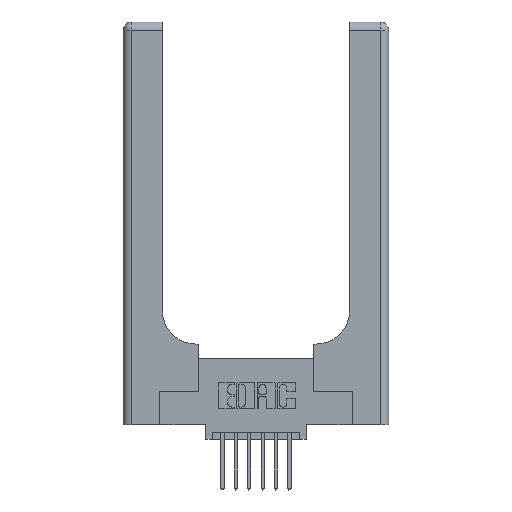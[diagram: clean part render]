
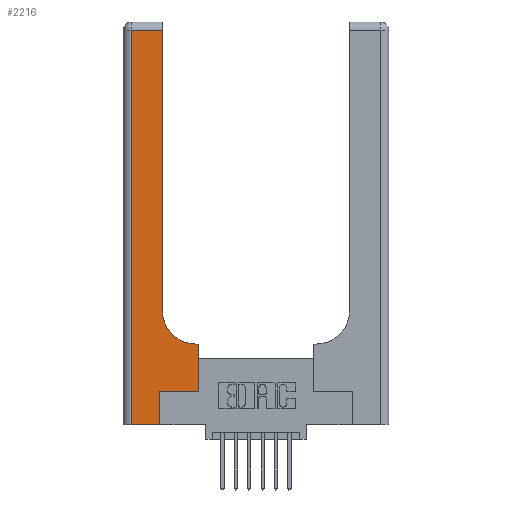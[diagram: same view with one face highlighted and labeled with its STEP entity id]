
A CAD part, top view. The second image highlights one B-rep face of the part: STEP entity #2216.
In plain terms, the highlighted planar face has unit normal (0, 0, 1).
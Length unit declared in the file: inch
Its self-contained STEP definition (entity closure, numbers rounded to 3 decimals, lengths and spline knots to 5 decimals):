
#297 = VECTOR ( 'NONE', #5770, 39.37008 ) ;
#603 = CARTESIAN_POINT ( 'NONE',  ( 0.269, 0., 0.37 ) ) ;
#843 = EDGE_CURVE ( 'NONE', #1696, #10269, #12274, .T. ) ;
#883 = AXIS2_PLACEMENT_3D ( 'NONE', #6288, #6208, #6057 ) ;
#1347 = LINE ( 'NONE', #8570, #10317 ) ;
#1508 = CARTESIAN_POINT ( 'NONE',  ( 0.2915, 0.6, 0.37 ) ) ;
#1696 = VERTEX_POINT ( 'NONE', #8972 ) ;
#1729 = CARTESIAN_POINT ( 'NONE',  ( 0.5415, 0.6, 0.37 ) ) ;
#2173 = AXIS2_PLACEMENT_3D ( 'NONE', #11557, #4662, #12651 ) ;
#2216 = ADVANCED_FACE ( 'NONE', ( #4907 ), #6676, .F. ) ;
#2738 = EDGE_CURVE ( 'NONE', #10291, #11556, #1347, .T. ) ;
#2952 = LINE ( 'NONE', #603, #14740 ) ;
#3196 = ORIENTED_EDGE ( 'NONE', *, *, #8487, .T. ) ;
#3889 = DIRECTION ( 'NONE',  ( -1., 0., 0. ) ) ;
#4345 = LINE ( 'NONE', #14715, #10156 ) ;
#4662 = DIRECTION ( 'NONE',  ( 0., 0., -1. ) ) ;
#4897 = ORIENTED_EDGE ( 'NONE', *, *, #2738, .T. ) ;
#4907 = FACE_OUTER_BOUND ( 'NONE', #8575, .T. ) ;
#5041 = VERTEX_POINT ( 'NONE', #7053 ) ;
#5174 = CARTESIAN_POINT ( 'NONE',  ( 0.5585, 0.6, 0.37 ) ) ;
#5247 = CIRCLE ( 'NONE', #2173, 0.25 ) ;
#5265 = VERTEX_POINT ( 'NONE', #5174 ) ;
#5685 = CARTESIAN_POINT ( 'NONE',  ( 0., 0., 0.37 ) ) ;
#5710 = VERTEX_POINT ( 'NONE', #5905 ) ;
#5770 = DIRECTION ( 'NONE',  ( 1., 0., 0. ) ) ;
#5905 = CARTESIAN_POINT ( 'NONE',  ( 0.2915, 0.85, 0.37 ) ) ;
#5964 = CARTESIAN_POINT ( 'NONE',  ( 0.269, 0., 0.37 ) ) ;
#5968 = DIRECTION ( 'NONE',  ( 0., -1., 0. ) ) ;
#6057 = DIRECTION ( 'NONE',  ( -1., 0., 0. ) ) ;
#6208 = DIRECTION ( 'NONE',  ( 0., 0., -1. ) ) ;
#6288 = CARTESIAN_POINT ( 'NONE',  ( 0., 3., 0.37 ) ) ;
#6676 = PLANE ( 'NONE',  #883 ) ;
#7053 = CARTESIAN_POINT ( 'NONE',  ( 0.06, 2.94, 0.37 ) ) ;
#7256 = VECTOR ( 'NONE', #8825, 39.37008 ) ;
#7663 = CARTESIAN_POINT ( 'NONE',  ( 0.2915, 3., 0.37 ) ) ;
#7739 = ORIENTED_EDGE ( 'NONE', *, *, #9788, .T. ) ;
#7916 = ORIENTED_EDGE ( 'NONE', *, *, #14826, .T. ) ;
#7942 = VECTOR ( 'NONE', #3889, 39.37008 ) ;
#7957 = VERTEX_POINT ( 'NONE', #14883 ) ;
#8397 = EDGE_CURVE ( 'NONE', #8807, #5710, #5247, .T. ) ;
#8431 = ORIENTED_EDGE ( 'NONE', *, *, #10467, .T. ) ;
#8487 = EDGE_CURVE ( 'NONE', #5041, #1696, #9951, .T. ) ;
#8570 = CARTESIAN_POINT ( 'NONE',  ( 0.269, 0.25, 0.37 ) ) ;
#8575 = EDGE_LOOP ( 'NONE', ( #9108, #7916, #3196, #12663, #8431, #4897, #10597, #7739, #14172 ) ) ;
#8655 = DIRECTION ( 'NONE',  ( 1., 0., 0. ) ) ;
#8807 = VERTEX_POINT ( 'NONE', #1729 ) ;
#8825 = DIRECTION ( 'NONE',  ( -1., 0., 0. ) ) ;
#8911 = LINE ( 'NONE', #7663, #11904 ) ;
#8972 = CARTESIAN_POINT ( 'NONE',  ( 0.06, 0., 0.37 ) ) ;
#9108 = ORIENTED_EDGE ( 'NONE', *, *, #14423, .T. ) ;
#9190 = DIRECTION ( 'NONE',  ( 0., 1., 0. ) ) ;
#9484 = CARTESIAN_POINT ( 'NONE',  ( 0.269, 0.25, 0.37 ) ) ;
#9597 = VECTOR ( 'NONE', #5968, 39.37008 ) ;
#9788 = EDGE_CURVE ( 'NONE', #5265, #8807, #11344, .T. ) ;
#9881 = CARTESIAN_POINT ( 'NONE',  ( 0.5585, 0.25, 0.37 ) ) ;
#9951 = LINE ( 'NONE', #13917, #9597 ) ;
#9963 = LINE ( 'NONE', #11129, #7256 ) ;
#10156 = VECTOR ( 'NONE', #9190, 39.37008 ) ;
#10269 = VERTEX_POINT ( 'NONE', #5964 ) ;
#10291 = VERTEX_POINT ( 'NONE', #9484 ) ;
#10317 = VECTOR ( 'NONE', #8655, 39.37008 ) ;
#10467 = EDGE_CURVE ( 'NONE', #10269, #10291, #2952, .T. ) ;
#10597 = ORIENTED_EDGE ( 'NONE', *, *, #14545, .T. ) ;
#11129 = CARTESIAN_POINT ( 'NONE',  ( 0., 2.94, 0.37 ) ) ;
#11344 = LINE ( 'NONE', #1508, #7942 ) ;
#11556 = VERTEX_POINT ( 'NONE', #9881 ) ;
#11557 = CARTESIAN_POINT ( 'NONE',  ( 0.5415, 0.85, 0.37 ) ) ;
#11904 = VECTOR ( 'NONE', #13300, 39.37008 ) ;
#12215 = DIRECTION ( 'NONE',  ( 0., 1., 0. ) ) ;
#12274 = LINE ( 'NONE', #5685, #297 ) ;
#12651 = DIRECTION ( 'NONE',  ( 1., 0., 0. ) ) ;
#12663 = ORIENTED_EDGE ( 'NONE', *, *, #843, .T. ) ;
#13300 = DIRECTION ( 'NONE',  ( 0., 1., 0. ) ) ;
#13917 = CARTESIAN_POINT ( 'NONE',  ( 0.06, 3., 0.37 ) ) ;
#14172 = ORIENTED_EDGE ( 'NONE', *, *, #8397, .T. ) ;
#14423 = EDGE_CURVE ( 'NONE', #5710, #7957, #8911, .T. ) ;
#14545 = EDGE_CURVE ( 'NONE', #11556, #5265, #4345, .T. ) ;
#14715 = CARTESIAN_POINT ( 'NONE',  ( 0.5585, 0.25, 0.37 ) ) ;
#14740 = VECTOR ( 'NONE', #12215, 39.37008 ) ;
#14826 = EDGE_CURVE ( 'NONE', #7957, #5041, #9963, .T. ) ;
#14883 = CARTESIAN_POINT ( 'NONE',  ( 0.2915, 2.94, 0.37 ) ) ;
